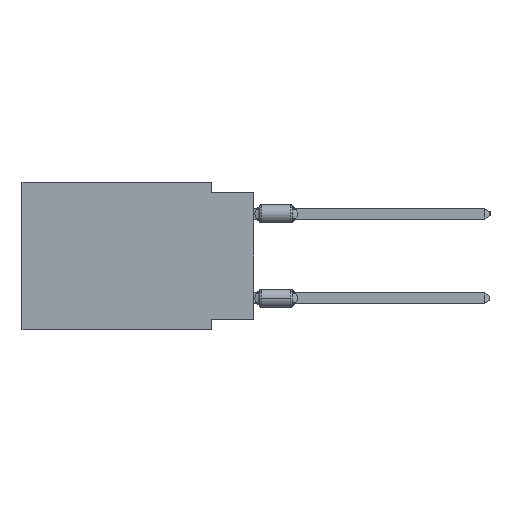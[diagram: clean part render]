
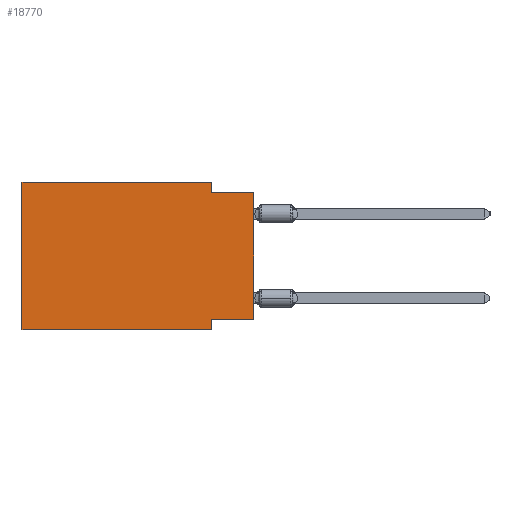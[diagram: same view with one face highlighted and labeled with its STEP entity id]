
A CAD part, left-side view. The second image highlights one B-rep face of the part: STEP entity #18770.
In plain terms, the highlighted planar face has unit normal (-1, 0, 0).
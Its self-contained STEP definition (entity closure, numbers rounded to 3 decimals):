
#488 = VERTEX_POINT ( 'NONE', #6549 ) ;
#799 = CARTESIAN_POINT ( 'NONE',  ( 0., 13.97, -8.89 ) ) ;
#1966 = VECTOR ( 'NONE', #40410, 1000. ) ;
#5526 = DIRECTION ( 'NONE',  ( 0., -1., 0. ) ) ;
#5782 = CARTESIAN_POINT ( 'NONE',  ( 0., 2.54, -8.255 ) ) ;
#6345 = CARTESIAN_POINT ( 'NONE',  ( 0., 13.97, -8.89 ) ) ;
#6549 = CARTESIAN_POINT ( 'NONE',  ( 0., 2.54, -8.89 ) ) ;
#6564 = LINE ( 'NONE', #12774, #1966 ) ;
#6839 = VECTOR ( 'NONE', #12496, 1000. ) ;
#7756 = EDGE_CURVE ( 'NONE', #22450, #11426, #39596, .T. ) ;
#8287 = CARTESIAN_POINT ( 'NONE',  ( 0., 0., 0. ) ) ;
#8475 = ORIENTED_EDGE ( 'NONE', *, *, #7756, .T. ) ;
#8724 = EDGE_CURVE ( 'NONE', #23371, #23564, #32718, .T. ) ;
#9143 = ORIENTED_EDGE ( 'NONE', *, *, #8724, .F. ) ;
#9632 = EDGE_CURVE ( 'NONE', #23564, #26636, #21871, .T. ) ;
#11024 = PLANE ( 'NONE',  #14561 ) ;
#11426 = VERTEX_POINT ( 'NONE', #22848 ) ;
#12239 = DIRECTION ( 'NONE',  ( 0., 0., -1. ) ) ;
#12478 = VECTOR ( 'NONE', #21537, 1000. ) ;
#12496 = DIRECTION ( 'NONE',  ( 0., -1., 0. ) ) ;
#12774 = CARTESIAN_POINT ( 'NONE',  ( 0., 13.97, 0. ) ) ;
#13604 = LINE ( 'NONE', #31388, #38957 ) ;
#14561 = AXIS2_PLACEMENT_3D ( 'NONE', #31577, #17427, #20635 ) ;
#14760 = DIRECTION ( 'NONE',  ( 0., -1., 0. ) ) ;
#15462 = VECTOR ( 'NONE', #5526, 1000. ) ;
#16048 = CARTESIAN_POINT ( 'NONE',  ( 0., 13.97, 0. ) ) ;
#17427 = DIRECTION ( 'NONE',  ( 1., 0., 0. ) ) ;
#18177 = LINE ( 'NONE', #799, #43064 ) ;
#18770 = ADVANCED_FACE ( 'NONE', ( #21303 ), #11024, .F. ) ;
#19088 = LINE ( 'NONE', #43534, #29209 ) ;
#19871 = EDGE_CURVE ( 'NONE', #39078, #488, #18177, .T. ) ;
#19977 = EDGE_CURVE ( 'NONE', #39660, #488, #19088, .T. ) ;
#20635 = DIRECTION ( 'NONE',  ( 0., 0., -1. ) ) ;
#21303 = FACE_OUTER_BOUND ( 'NONE', #44132, .T. ) ;
#21537 = DIRECTION ( 'NONE',  ( 0., 0., 1. ) ) ;
#21871 = LINE ( 'NONE', #35818, #26166 ) ;
#22357 = EDGE_CURVE ( 'NONE', #39078, #23371, #6564, .T. ) ;
#22450 = VERTEX_POINT ( 'NONE', #39438 ) ;
#22848 = CARTESIAN_POINT ( 'NONE',  ( 0., 0., -0.635 ) ) ;
#22988 = LINE ( 'NONE', #29841, #6839 ) ;
#23371 = VERTEX_POINT ( 'NONE', #36762 ) ;
#23564 = VERTEX_POINT ( 'NONE', #41529 ) ;
#23925 = EDGE_CURVE ( 'NONE', #26636, #11426, #22988, .T. ) ;
#24929 = ORIENTED_EDGE ( 'NONE', *, *, #19977, .F. ) ;
#26166 = VECTOR ( 'NONE', #33299, 1000. ) ;
#26636 = VERTEX_POINT ( 'NONE', #29354 ) ;
#27311 = ORIENTED_EDGE ( 'NONE', *, *, #22357, .F. ) ;
#27525 = DIRECTION ( 'NONE',  ( 0., 1., 0. ) ) ;
#28999 = ORIENTED_EDGE ( 'NONE', *, *, #9632, .F. ) ;
#29054 = ORIENTED_EDGE ( 'NONE', *, *, #23925, .F. ) ;
#29209 = VECTOR ( 'NONE', #12239, 1000. ) ;
#29354 = CARTESIAN_POINT ( 'NONE',  ( 0., 2.54, -0.635 ) ) ;
#29701 = ORIENTED_EDGE ( 'NONE', *, *, #39418, .F. ) ;
#29841 = CARTESIAN_POINT ( 'NONE',  ( 0., 0., -0.635 ) ) ;
#31388 = CARTESIAN_POINT ( 'NONE',  ( 0., 0., -8.255 ) ) ;
#31577 = CARTESIAN_POINT ( 'NONE',  ( 0., 13.97, 0. ) ) ;
#32718 = LINE ( 'NONE', #16048, #15462 ) ;
#33299 = DIRECTION ( 'NONE',  ( 0., 0., -1. ) ) ;
#35818 = CARTESIAN_POINT ( 'NONE',  ( 0., 2.54, 0. ) ) ;
#36762 = CARTESIAN_POINT ( 'NONE',  ( 0., 13.97, 0. ) ) ;
#38957 = VECTOR ( 'NONE', #27525, 1000. ) ;
#39078 = VERTEX_POINT ( 'NONE', #6345 ) ;
#39418 = EDGE_CURVE ( 'NONE', #22450, #39660, #13604, .T. ) ;
#39438 = CARTESIAN_POINT ( 'NONE',  ( 0., 0., -8.255 ) ) ;
#39596 = LINE ( 'NONE', #8287, #12478 ) ;
#39660 = VERTEX_POINT ( 'NONE', #5782 ) ;
#40410 = DIRECTION ( 'NONE',  ( 0., 0., 1. ) ) ;
#40699 = ORIENTED_EDGE ( 'NONE', *, *, #19871, .T. ) ;
#41529 = CARTESIAN_POINT ( 'NONE',  ( 0., 2.54, 0. ) ) ;
#43064 = VECTOR ( 'NONE', #14760, 1000. ) ;
#43534 = CARTESIAN_POINT ( 'NONE',  ( 0., 2.54, -8.89 ) ) ;
#44132 = EDGE_LOOP ( 'NONE', ( #8475, #29054, #28999, #9143, #27311, #40699, #24929, #29701 ) ) ;
